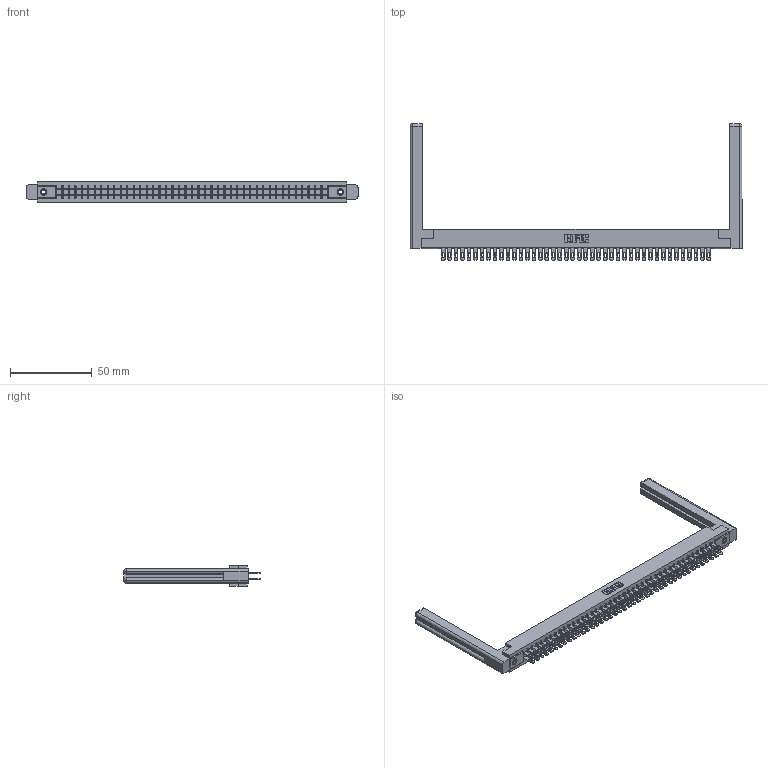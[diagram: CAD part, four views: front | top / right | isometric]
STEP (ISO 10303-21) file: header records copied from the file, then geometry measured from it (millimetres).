
FILE_DESCRIPTION (( 'STEP AP203' ), '1' );
FILE_NAME ('355-084-500-558.STEP', '2019-09-13T15:45:58', ( '' ), ( '' ), 'SwSTEP 2.0', 'SolidWorks 2016', '' );
FILE_SCHEMA (( 'CONFIG_CONTROL_DESIGN' ));
Length unit declared in the file: inch
Products named in the file (5): 305-290-001_500; 345-250-001_345-250-001-102; 307-220-058; 305 Part_.156 Dia; 355-084-500-558
Assembly tree (89 placements, depth 2):
  355-084-500-558
    305 Part_.156 Dia
    305-290-001_500  x84
    345-250-001_345-250-001-102  x2
    307-220-058  x2
Bounding box: 203.05 x 83.49 x 12.7 mm (x, y, z)
Volume: 28018.8 mm3; surface area: 33972.8 mm2
Topology: 89 solids, 89 shells, 4458 faces, 12724 edges, 8244 vertices
Faces by surface type: plane 2504, cylinder 1762, sphere 168, cone 12, torus 12
Entity records: 48130 total; most frequent: CARTESIAN_POINT 7979, ORIENTED_EDGE 7862, DIRECTION 7683, EDGE_CURVE 3931, VECTOR 3167, LINE 3167, VERTEX_POINT 2500, AXIS2_PLACEMENT_3D 2258
